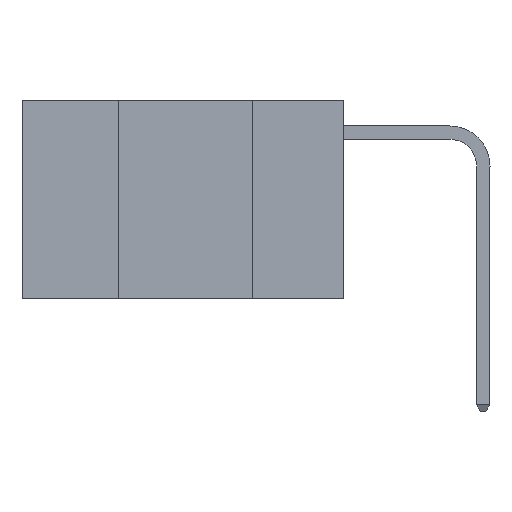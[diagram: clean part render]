
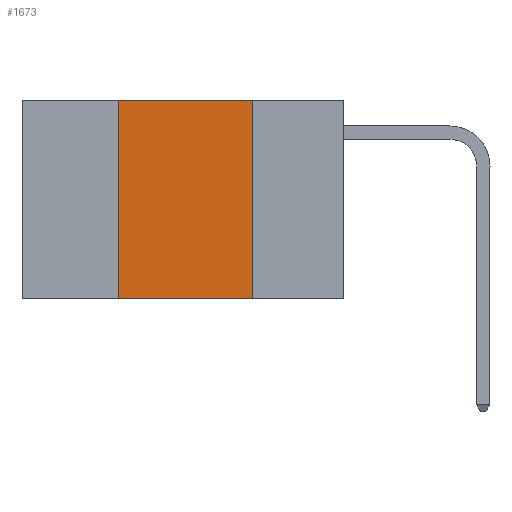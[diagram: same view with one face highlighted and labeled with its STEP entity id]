
A CAD part, left-side view. The second image highlights one B-rep face of the part: STEP entity #1673.
In plain terms, the highlighted planar face has unit normal (-1, 0, 0).
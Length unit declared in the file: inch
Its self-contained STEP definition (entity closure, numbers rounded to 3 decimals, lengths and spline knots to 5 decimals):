
#274 = DIRECTION ( 'NONE',  ( 0., -1., 0. ) ) ;
#500 = ORIENTED_EDGE ( 'NONE', *, *, #4412, .T. ) ;
#1202 = DIRECTION ( 'NONE',  ( 0., 0., 1. ) ) ;
#1239 = CARTESIAN_POINT ( 'NONE',  ( 0., 0.17, 0. ) ) ;
#1271 = LINE ( 'NONE', #10279, #7536 ) ;
#1301 = VERTEX_POINT ( 'NONE', #8709 ) ;
#1392 = LINE ( 'NONE', #10073, #13911 ) ;
#1575 = CARTESIAN_POINT ( 'NONE',  ( 0., 0.42, -0.37 ) ) ;
#1577 = CARTESIAN_POINT ( 'NONE',  ( 0., 0.6, -0.37 ) ) ;
#1673 = ADVANCED_FACE ( 'NONE', ( #12124 ), #4746, .F. ) ;
#1803 = VERTEX_POINT ( 'NONE', #13816 ) ;
#2562 = EDGE_LOOP ( 'NONE', ( #3076, #3481, #13052, #500 ) ) ;
#2998 = EDGE_CURVE ( 'NONE', #10466, #1803, #12373, .T. ) ;
#3076 = ORIENTED_EDGE ( 'NONE', *, *, #4555, .F. ) ;
#3481 = ORIENTED_EDGE ( 'NONE', *, *, #5953, .F. ) ;
#4071 = VECTOR ( 'NONE', #8969, 39.37008 ) ;
#4412 = EDGE_CURVE ( 'NONE', #10466, #1301, #7350, .T. ) ;
#4555 = EDGE_CURVE ( 'NONE', #13616, #1301, #1271, .T. ) ;
#4746 = PLANE ( 'NONE',  #7444 ) ;
#4822 = DIRECTION ( 'NONE',  ( 0., 0., -1. ) ) ;
#5953 = EDGE_CURVE ( 'NONE', #1803, #13616, #1392, .T. ) ;
#6131 = VECTOR ( 'NONE', #1202, 39.37008 ) ;
#7350 = LINE ( 'NONE', #1577, #4071 ) ;
#7444 = AXIS2_PLACEMENT_3D ( 'NONE', #12662, #15245, #4822 ) ;
#7536 = VECTOR ( 'NONE', #15018, 39.37008 ) ;
#8709 = CARTESIAN_POINT ( 'NONE',  ( 0., 0.17, -0.37 ) ) ;
#8969 = DIRECTION ( 'NONE',  ( 0., -1., 0. ) ) ;
#10073 = CARTESIAN_POINT ( 'NONE',  ( 0., 0.6, 0. ) ) ;
#10279 = CARTESIAN_POINT ( 'NONE',  ( 0., 0.17, 0. ) ) ;
#10466 = VERTEX_POINT ( 'NONE', #1575 ) ;
#12104 = CARTESIAN_POINT ( 'NONE',  ( 0., 0.42, 0. ) ) ;
#12124 = FACE_OUTER_BOUND ( 'NONE', #2562, .T. ) ;
#12373 = LINE ( 'NONE', #12104, #6131 ) ;
#12662 = CARTESIAN_POINT ( 'NONE',  ( 0., 0.6, 0. ) ) ;
#13052 = ORIENTED_EDGE ( 'NONE', *, *, #2998, .F. ) ;
#13616 = VERTEX_POINT ( 'NONE', #1239 ) ;
#13816 = CARTESIAN_POINT ( 'NONE',  ( 0., 0.42, 0. ) ) ;
#13911 = VECTOR ( 'NONE', #274, 39.37008 ) ;
#15018 = DIRECTION ( 'NONE',  ( 0., 0., -1. ) ) ;
#15245 = DIRECTION ( 'NONE',  ( 1., 0., 0. ) ) ;
